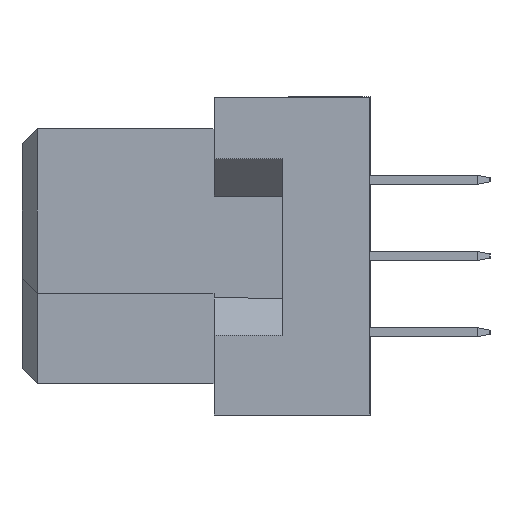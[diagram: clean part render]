
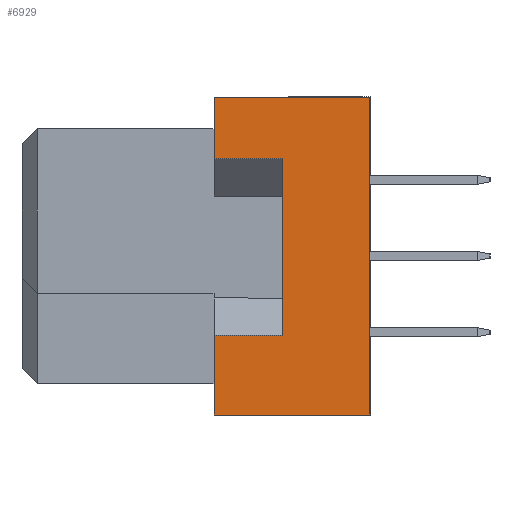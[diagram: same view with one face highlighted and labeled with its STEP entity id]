
A CAD part, left-side view. The second image highlights one B-rep face of the part: STEP entity #6929.
In plain terms, the highlighted planar face has unit normal (-1, 0, 0).
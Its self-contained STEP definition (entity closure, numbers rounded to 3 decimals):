
#96 = CARTESIAN_POINT ( 'NONE',  ( -27.5, -8.7, 3.25 ) ) ;
#217 = FACE_OUTER_BOUND ( 'NONE', #5818, .T. ) ;
#518 = VECTOR ( 'NONE', #16619, 1000. ) ;
#1288 = DIRECTION ( 'NONE',  ( 0., 1., 0. ) ) ;
#1290 = LINE ( 'NONE', #4311, #15152 ) ;
#1745 = EDGE_CURVE ( 'NONE', #2313, #6372, #17499, .T. ) ;
#2313 = VERTEX_POINT ( 'NONE', #6742 ) ;
#2378 = VERTEX_POINT ( 'NONE', #8597 ) ;
#2423 = EDGE_CURVE ( 'NONE', #2313, #8265, #4264, .T. ) ;
#2722 = CARTESIAN_POINT ( 'NONE',  ( -27.5, -11.6, -5.3 ) ) ;
#2736 = ORIENTED_EDGE ( 'NONE', *, *, #14134, .F. ) ;
#2911 = ORIENTED_EDGE ( 'NONE', *, *, #4400, .F. ) ;
#3363 = DIRECTION ( 'NONE',  ( -1., 0., 0. ) ) ;
#3574 = CARTESIAN_POINT ( 'NONE',  ( -27.5, -8.7, -2.65 ) ) ;
#4264 = LINE ( 'NONE', #12564, #10020 ) ;
#4283 = CARTESIAN_POINT ( 'NONE',  ( -27.5, -8.7, -2.65 ) ) ;
#4311 = CARTESIAN_POINT ( 'NONE',  ( -27.5, -6.4, -5.3 ) ) ;
#4345 = CARTESIAN_POINT ( 'NONE',  ( -27.5, -6.4, 5.3 ) ) ;
#4400 = EDGE_CURVE ( 'NONE', #10163, #16800, #12767, .T. ) ;
#4536 = EDGE_CURVE ( 'NONE', #2378, #18890, #16943, .T. ) ;
#4887 = DIRECTION ( 'NONE',  ( 0., 0., 1. ) ) ;
#4919 = VERTEX_POINT ( 'NONE', #96 ) ;
#5818 = EDGE_LOOP ( 'NONE', ( #7917, #16675, #15941, #9872, #6162, #2911, #2736, #7919 ) ) ;
#6162 = ORIENTED_EDGE ( 'NONE', *, *, #15412, .T. ) ;
#6372 = VERTEX_POINT ( 'NONE', #14272 ) ;
#6742 = CARTESIAN_POINT ( 'NONE',  ( -27.5, -11.6, -5.3 ) ) ;
#6929 = ADVANCED_FACE ( 'NONE', ( #217 ), #8422, .T. ) ;
#7917 = ORIENTED_EDGE ( 'NONE', *, *, #4536, .T. ) ;
#7919 = ORIENTED_EDGE ( 'NONE', *, *, #14588, .F. ) ;
#8265 = VERTEX_POINT ( 'NONE', #11464 ) ;
#8422 = PLANE ( 'NONE',  #17366 ) ;
#8597 = CARTESIAN_POINT ( 'NONE',  ( -27.5, -8.7, -2.65 ) ) ;
#9211 = VECTOR ( 'NONE', #17905, 1000. ) ;
#9309 = DIRECTION ( 'NONE',  ( 0., 1., 0. ) ) ;
#9362 = VECTOR ( 'NONE', #9309, 1000. ) ;
#9418 = CARTESIAN_POINT ( 'NONE',  ( -27.5, -6.4, -5.3 ) ) ;
#9872 = ORIENTED_EDGE ( 'NONE', *, *, #2423, .T. ) ;
#10020 = VECTOR ( 'NONE', #17408, 1000. ) ;
#10163 = VERTEX_POINT ( 'NONE', #18022 ) ;
#10466 = EDGE_CURVE ( 'NONE', #6372, #18890, #1290, .T. ) ;
#10788 = CARTESIAN_POINT ( 'NONE',  ( -27.5, -8.7, 3.25 ) ) ;
#10924 = LINE ( 'NONE', #17376, #9211 ) ;
#11464 = CARTESIAN_POINT ( 'NONE',  ( -27.5, -11.6, 5.3 ) ) ;
#12289 = VECTOR ( 'NONE', #1288, 1000. ) ;
#12564 = CARTESIAN_POINT ( 'NONE',  ( -27.5, -11.6, 5.3 ) ) ;
#12767 = LINE ( 'NONE', #9418, #17397 ) ;
#14134 = EDGE_CURVE ( 'NONE', #4919, #10163, #17348, .T. ) ;
#14255 = DIRECTION ( 'NONE',  ( 0., 0., 1. ) ) ;
#14272 = CARTESIAN_POINT ( 'NONE',  ( -27.5, -6.4, -5.3 ) ) ;
#14588 = EDGE_CURVE ( 'NONE', #2378, #4919, #19153, .T. ) ;
#15152 = VECTOR ( 'NONE', #21026, 1000. ) ;
#15412 = EDGE_CURVE ( 'NONE', #8265, #16800, #10924, .T. ) ;
#15941 = ORIENTED_EDGE ( 'NONE', *, *, #1745, .F. ) ;
#16619 = DIRECTION ( 'NONE',  ( 0., 1., 0. ) ) ;
#16675 = ORIENTED_EDGE ( 'NONE', *, *, #10466, .F. ) ;
#16770 = CARTESIAN_POINT ( 'NONE',  ( -27.5, -6.4, -2.65 ) ) ;
#16800 = VERTEX_POINT ( 'NONE', #4345 ) ;
#16943 = LINE ( 'NONE', #3574, #518 ) ;
#17348 = LINE ( 'NONE', #10788, #12289 ) ;
#17366 = AXIS2_PLACEMENT_3D ( 'NONE', #19648, #3363, #4887 ) ;
#17376 = CARTESIAN_POINT ( 'NONE',  ( -27.5, -11.6, 5.3 ) ) ;
#17397 = VECTOR ( 'NONE', #14255, 1000. ) ;
#17408 = DIRECTION ( 'NONE',  ( 0., 0., 1. ) ) ;
#17499 = LINE ( 'NONE', #2722, #9362 ) ;
#17905 = DIRECTION ( 'NONE',  ( 0., 1., 0. ) ) ;
#18022 = CARTESIAN_POINT ( 'NONE',  ( -27.5, -6.4, 3.25 ) ) ;
#18890 = VERTEX_POINT ( 'NONE', #16770 ) ;
#19153 = LINE ( 'NONE', #4283, #20212 ) ;
#19648 = CARTESIAN_POINT ( 'NONE',  ( -27.5, -11.6, 5.3 ) ) ;
#20212 = VECTOR ( 'NONE', #20991, 1000. ) ;
#20991 = DIRECTION ( 'NONE',  ( 0., 0., 1. ) ) ;
#21026 = DIRECTION ( 'NONE',  ( 0., 0., 1. ) ) ;
